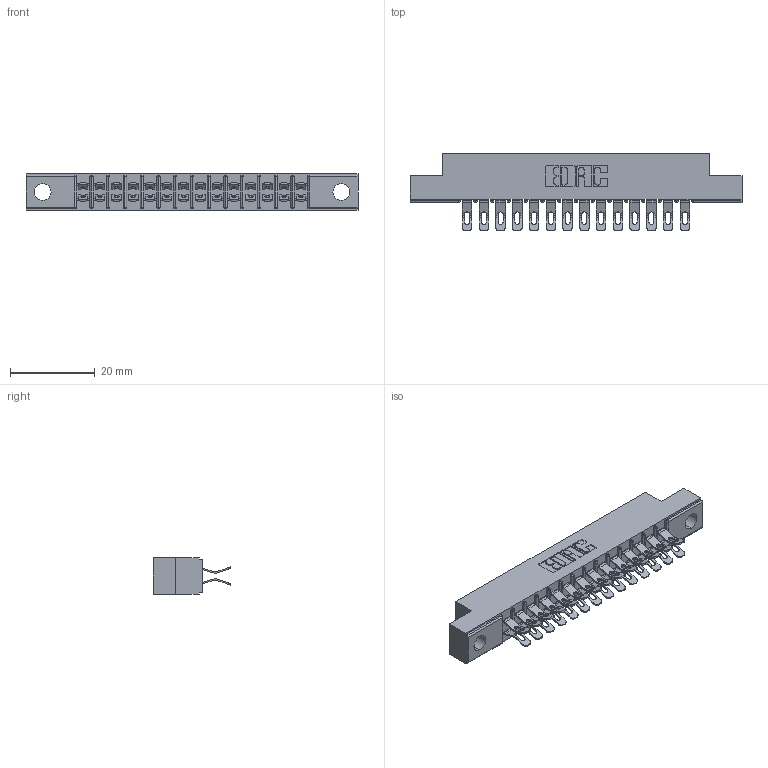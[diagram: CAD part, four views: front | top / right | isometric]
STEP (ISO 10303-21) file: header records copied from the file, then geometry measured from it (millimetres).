
FILE_DESCRIPTION (( 'STEP AP203' ), '1' );
FILE_NAME ('315-028-555-204.STEP', '2019-09-10T15:12:08', ( '' ), ( '' ), 'SwSTEP 2.0', 'SolidWorks 2016', '' );
FILE_SCHEMA (( 'CONFIG_CONTROL_DESIGN' ));
Length unit declared in the file: inch
Products named in the file (3): 305-290-001_555; 305 Part_.156 Dia; 315-028-555-204
Assembly tree (29 placements, depth 2):
  315-028-555-204
    305 Part_.156 Dia
    305-290-001_555  x28
Bounding box: 78.49 x 18.41 x 8.71 mm (x, y, z)
Volume: 4915.3 mm3; surface area: 9176.8 mm2
Topology: 29 solids, 29 shells, 1978 faces, 5882 edges, 3844 vertices
Faces by surface type: plane 978, cylinder 944, sphere 56
Entity records: 19609 total; most frequent: CARTESIAN_POINT 3268, ORIENTED_EDGE 3228, DIRECTION 3170, EDGE_CURVE 1614, LINE 1262, VECTOR 1262, VERTEX_POINT 1036, AXIS2_PLACEMENT_3D 954
